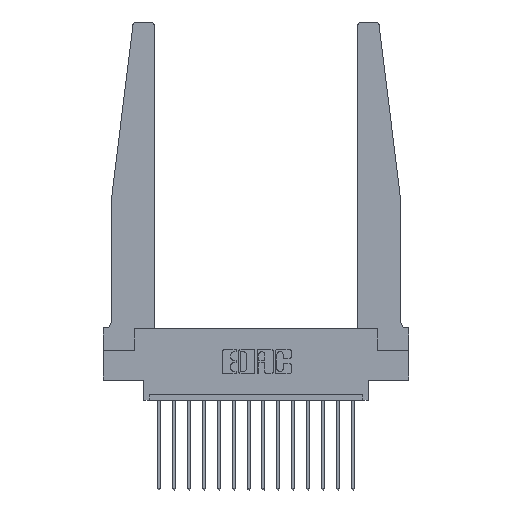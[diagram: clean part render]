
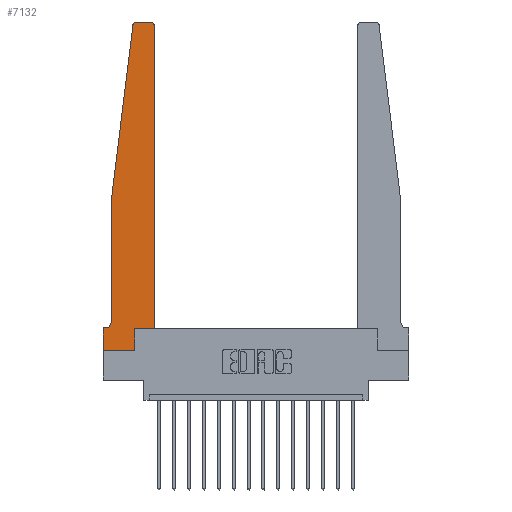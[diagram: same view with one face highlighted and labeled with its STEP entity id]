
A CAD part, top view. The second image highlights one B-rep face of the part: STEP entity #7132.
In plain terms, the highlighted planar face has unit normal (0, 0, 1).
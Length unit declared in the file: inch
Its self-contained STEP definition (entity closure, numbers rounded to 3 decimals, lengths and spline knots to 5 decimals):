
#73 = EDGE_CURVE ( 'NONE', #8571, #11590, #13114, .T. ) ;
#211 = ORIENTED_EDGE ( 'NONE', *, *, #11176, .T. ) ;
#371 = DIRECTION ( 'NONE',  ( -1., 0., 0. ) ) ;
#503 = CARTESIAN_POINT ( 'NONE',  ( 0., 0.1875, 0.37 ) ) ;
#1190 = DIRECTION ( 'NONE',  ( 0., -1., 0. ) ) ;
#1477 = AXIS2_PLACEMENT_3D ( 'NONE', #17295, #12976, #2141 ) ;
#1777 = VECTOR ( 'NONE', #11335, 39.37008 ) ;
#1884 = VERTEX_POINT ( 'NONE', #9605 ) ;
#1963 = ORIENTED_EDGE ( 'NONE', *, *, #15475, .T. ) ;
#2141 = DIRECTION ( 'NONE',  ( 1., 0., 0. ) ) ;
#2146 = LINE ( 'NONE', #17300, #10674 ) ;
#2392 = VERTEX_POINT ( 'NONE', #2901 ) ;
#2536 = VECTOR ( 'NONE', #10046, 39.37008 ) ;
#2547 = EDGE_CURVE ( 'NONE', #13950, #12452, #4719, .T. ) ;
#2800 = ORIENTED_EDGE ( 'NONE', *, *, #10594, .T. ) ;
#2901 = CARTESIAN_POINT ( 'NONE',  ( 0.065, 0.2375, 0.37 ) ) ;
#3008 = CARTESIAN_POINT ( 'NONE',  ( 0.065, 1.25, 0.37 ) ) ;
#3012 = EDGE_CURVE ( 'NONE', #2392, #10610, #7340, .T. ) ;
#3146 = CARTESIAN_POINT ( 'NONE',  ( 0.015, 0.2375, 0.37 ) ) ;
#3367 = VECTOR ( 'NONE', #7218, 39.37008 ) ;
#3588 = ORIENTED_EDGE ( 'NONE', *, *, #12286, .T. ) ;
#3862 = AXIS2_PLACEMENT_3D ( 'NONE', #3146, #8754, #371 ) ;
#3920 = VERTEX_POINT ( 'NONE', #15189 ) ;
#4071 = LINE ( 'NONE', #3008, #16171 ) ;
#4375 = DIRECTION ( 'NONE',  ( 1., 0., 0. ) ) ;
#4546 = ORIENTED_EDGE ( 'NONE', *, *, #13285, .T. ) ;
#4649 = CIRCLE ( 'NONE', #11542, 0.03 ) ;
#4714 = DIRECTION ( 'NONE',  ( -1., 0., 0. ) ) ;
#4719 = LINE ( 'NONE', #10281, #15341 ) ;
#4842 = EDGE_CURVE ( 'NONE', #8361, #12050, #11458, .T. ) ;
#4926 = VERTEX_POINT ( 'NONE', #11974 ) ;
#5170 = CARTESIAN_POINT ( 'NONE',  ( 0., 0.1875, 0.37 ) ) ;
#5607 = ORIENTED_EDGE ( 'NONE', *, *, #2547, .T. ) ;
#5852 = DIRECTION ( 'NONE',  ( 1., 0., 0. ) ) ;
#5854 = CARTESIAN_POINT ( 'NONE',  ( 0., 0., 0.37 ) ) ;
#6147 = ORIENTED_EDGE ( 'NONE', *, *, #3012, .T. ) ;
#6547 = ORIENTED_EDGE ( 'NONE', *, *, #73, .T. ) ;
#6576 = VECTOR ( 'NONE', #13201, 39.37008 ) ;
#7027 = DIRECTION ( 'NONE',  ( 1., 0., 0. ) ) ;
#7132 = ADVANCED_FACE ( 'NONE', ( #16886 ), #13991, .T. ) ;
#7150 = LINE ( 'NONE', #10207, #2536 ) ;
#7161 = ORIENTED_EDGE ( 'NONE', *, *, #15487, .T. ) ;
#7182 = CARTESIAN_POINT ( 'NONE',  ( 0.27653, 2.72, 0.37 ) ) ;
#7218 = DIRECTION ( 'NONE',  ( 0., 1., 0. ) ) ;
#7335 = CARTESIAN_POINT ( 'NONE',  ( 0., 0., 0.37 ) ) ;
#7340 = CIRCLE ( 'NONE', #3862, 0.05 ) ;
#8361 = VERTEX_POINT ( 'NONE', #15357 ) ;
#8429 = LINE ( 'NONE', #15340, #15620 ) ;
#8555 = CARTESIAN_POINT ( 'NONE',  ( 0.395, 2.75, 0.37 ) ) ;
#8571 = VERTEX_POINT ( 'NONE', #5170 ) ;
#8754 = DIRECTION ( 'NONE',  ( 0., 0., -1. ) ) ;
#8948 = CARTESIAN_POINT ( 'NONE',  ( 0.2605, 0.18, 0.37 ) ) ;
#9033 = EDGE_LOOP ( 'NONE', ( #1963, #211, #11808, #7161, #6147, #4546, #6547, #3588, #13673, #2800, #5607, #14982 ) ) ;
#9266 = CIRCLE ( 'NONE', #1477, 0.03 ) ;
#9605 = CARTESIAN_POINT ( 'NONE',  ( 0.27653, 2.75, 0.37 ) ) ;
#9624 = CARTESIAN_POINT ( 'NONE',  ( 0.425, 0.18, 0.37 ) ) ;
#9870 = EDGE_CURVE ( 'NONE', #3920, #4926, #7150, .T. ) ;
#10046 = DIRECTION ( 'NONE',  ( -0.122, -0.992, 0. ) ) ;
#10207 = CARTESIAN_POINT ( 'NONE',  ( 0.065, 1.25, 0.37 ) ) ;
#10281 = CARTESIAN_POINT ( 'NONE',  ( 0.425, 0.18, 0.37 ) ) ;
#10594 = EDGE_CURVE ( 'NONE', #12050, #13950, #13755, .T. ) ;
#10610 = VERTEX_POINT ( 'NONE', #14915 ) ;
#10674 = VECTOR ( 'NONE', #4714, 39.37008 ) ;
#11176 = EDGE_CURVE ( 'NONE', #1884, #3920, #4649, .T. ) ;
#11335 = DIRECTION ( 'NONE',  ( 1., 0., 0. ) ) ;
#11458 = LINE ( 'NONE', #16938, #3367 ) ;
#11542 = AXIS2_PLACEMENT_3D ( 'NONE', #7182, #12669, #5852 ) ;
#11583 = LINE ( 'NONE', #5854, #1777 ) ;
#11590 = VERTEX_POINT ( 'NONE', #7335 ) ;
#11808 = ORIENTED_EDGE ( 'NONE', *, *, #9870, .T. ) ;
#11974 = CARTESIAN_POINT ( 'NONE',  ( 0.065, 1.25, 0.37 ) ) ;
#12050 = VERTEX_POINT ( 'NONE', #8948 ) ;
#12076 = EDGE_CURVE ( 'NONE', #12452, #12270, #9266, .T. ) ;
#12270 = VERTEX_POINT ( 'NONE', #8555 ) ;
#12286 = EDGE_CURVE ( 'NONE', #11590, #8361, #11583, .T. ) ;
#12452 = VERTEX_POINT ( 'NONE', #15972 ) ;
#12669 = DIRECTION ( 'NONE',  ( 0., 0., 1. ) ) ;
#12868 = AXIS2_PLACEMENT_3D ( 'NONE', #503, #12916, #4375 ) ;
#12916 = DIRECTION ( 'NONE',  ( 0., 0., 1. ) ) ;
#12950 = VECTOR ( 'NONE', #7027, 39.37008 ) ;
#12976 = DIRECTION ( 'NONE',  ( 0., 0., 1. ) ) ;
#13114 = LINE ( 'NONE', #14546, #6576 ) ;
#13201 = DIRECTION ( 'NONE',  ( 0., -1., 0. ) ) ;
#13285 = EDGE_CURVE ( 'NONE', #10610, #8571, #2146, .T. ) ;
#13666 = CARTESIAN_POINT ( 'NONE',  ( 0.425, 0.18, 0.37 ) ) ;
#13673 = ORIENTED_EDGE ( 'NONE', *, *, #4842, .T. ) ;
#13755 = LINE ( 'NONE', #13666, #12950 ) ;
#13950 = VERTEX_POINT ( 'NONE', #9624 ) ;
#13991 = PLANE ( 'NONE',  #12868 ) ;
#14414 = DIRECTION ( 'NONE',  ( 0., 1., 0. ) ) ;
#14546 = CARTESIAN_POINT ( 'NONE',  ( 0., 0., 0.37 ) ) ;
#14915 = CARTESIAN_POINT ( 'NONE',  ( 0.015, 0.1875, 0.37 ) ) ;
#14982 = ORIENTED_EDGE ( 'NONE', *, *, #12076, .T. ) ;
#15189 = CARTESIAN_POINT ( 'NONE',  ( 0.24675, 2.72367, 0.37 ) ) ;
#15248 = DIRECTION ( 'NONE',  ( -1., 0., 0. ) ) ;
#15341 = VECTOR ( 'NONE', #14414, 39.37008 ) ;
#15340 = CARTESIAN_POINT ( 'NONE',  ( 0.25, 2.75, 0.37 ) ) ;
#15357 = CARTESIAN_POINT ( 'NONE',  ( 0.2605, 0., 0.37 ) ) ;
#15475 = EDGE_CURVE ( 'NONE', #12270, #1884, #8429, .T. ) ;
#15487 = EDGE_CURVE ( 'NONE', #4926, #2392, #4071, .T. ) ;
#15620 = VECTOR ( 'NONE', #15248, 39.37008 ) ;
#15972 = CARTESIAN_POINT ( 'NONE',  ( 0.425, 2.72, 0.37 ) ) ;
#16171 = VECTOR ( 'NONE', #1190, 39.37008 ) ;
#16886 = FACE_OUTER_BOUND ( 'NONE', #9033, .T. ) ;
#16938 = CARTESIAN_POINT ( 'NONE',  ( 0.2605, 0.18, 0.37 ) ) ;
#17295 = CARTESIAN_POINT ( 'NONE',  ( 0.395, 2.72, 0.37 ) ) ;
#17300 = CARTESIAN_POINT ( 'NONE',  ( 0.065, 0.1875, 0.37 ) ) ;
